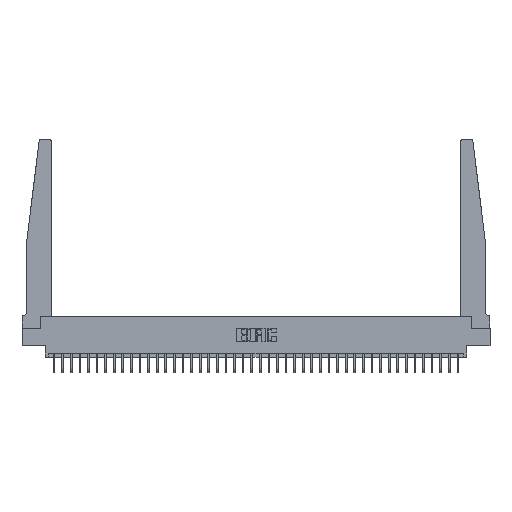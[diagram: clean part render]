
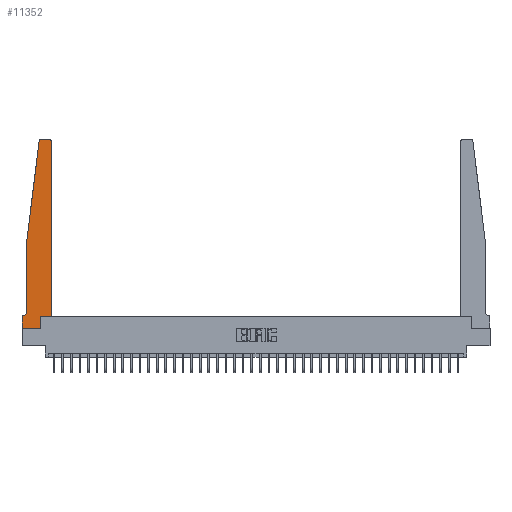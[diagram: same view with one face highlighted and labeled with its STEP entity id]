
A CAD part, top view. The second image highlights one B-rep face of the part: STEP entity #11352.
In plain terms, the highlighted planar face has unit normal (0, 0, 1).
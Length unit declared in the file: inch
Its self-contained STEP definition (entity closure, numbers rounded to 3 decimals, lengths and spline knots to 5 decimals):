
#460 = CARTESIAN_POINT ( 'NONE',  ( 0.425, 2.72, 0.37 ) ) ;
#1058 = EDGE_LOOP ( 'NONE', ( #14955, #33031, #28609, #17216, #21894, #33223, #4994, #19505, #8686, #12310, #12624, #16749 ) ) ;
#1568 = VERTEX_POINT ( 'NONE', #8934 ) ;
#1722 = LINE ( 'NONE', #28738, #21538 ) ;
#2375 = DIRECTION ( 'NONE',  ( 1., 0., 0. ) ) ;
#2389 = LINE ( 'NONE', #35909, #11811 ) ;
#3018 = CARTESIAN_POINT ( 'NONE',  ( 0.24675, 2.72367, 0.37 ) ) ;
#3846 = CARTESIAN_POINT ( 'NONE',  ( 0.015, 0.2375, 0.37 ) ) ;
#4205 = VECTOR ( 'NONE', #15173, 39.37008 ) ;
#4994 = ORIENTED_EDGE ( 'NONE', *, *, #14231, .T. ) ;
#5200 = VERTEX_POINT ( 'NONE', #8440 ) ;
#6178 = AXIS2_PLACEMENT_3D ( 'NONE', #28668, #14218, #34737 ) ;
#6329 = DIRECTION ( 'NONE',  ( 0., 1., 0. ) ) ;
#6392 = EDGE_CURVE ( 'NONE', #35005, #17127, #34311, .T. ) ;
#6412 = DIRECTION ( 'NONE',  ( 1., 0., 0. ) ) ;
#6859 = PLANE ( 'NONE',  #18879 ) ;
#7048 = DIRECTION ( 'NONE',  ( -1., 0., 0. ) ) ;
#7368 = DIRECTION ( 'NONE',  ( -0.122, -0.992, 0. ) ) ;
#7501 = CARTESIAN_POINT ( 'NONE',  ( 0.2605, 0., 0.37 ) ) ;
#7635 = EDGE_CURVE ( 'NONE', #17127, #5200, #26704, .T. ) ;
#7813 = VERTEX_POINT ( 'NONE', #18453 ) ;
#7896 = DIRECTION ( 'NONE',  ( 1., 0., 0. ) ) ;
#7900 = VERTEX_POINT ( 'NONE', #30471 ) ;
#8000 = DIRECTION ( 'NONE',  ( 0., 0., 1. ) ) ;
#8421 = VERTEX_POINT ( 'NONE', #22709 ) ;
#8440 = CARTESIAN_POINT ( 'NONE',  ( 0.2605, 0.18, 0.37 ) ) ;
#8665 = CIRCLE ( 'NONE', #6178, 0.03 ) ;
#8686 = ORIENTED_EDGE ( 'NONE', *, *, #7635, .T. ) ;
#8934 = CARTESIAN_POINT ( 'NONE',  ( 0.065, 1.25, 0.37 ) ) ;
#9943 = CARTESIAN_POINT ( 'NONE',  ( 0.425, 0.18, 0.37 ) ) ;
#10361 = DIRECTION ( 'NONE',  ( -1., 0., 0. ) ) ;
#11352 = ADVANCED_FACE ( 'NONE', ( #17073 ), #6859, .T. ) ;
#11811 = VECTOR ( 'NONE', #36038, 39.37008 ) ;
#12098 = CARTESIAN_POINT ( 'NONE',  ( 0.2605, 0.18, 0.37 ) ) ;
#12310 = ORIENTED_EDGE ( 'NONE', *, *, #14349, .T. ) ;
#12624 = ORIENTED_EDGE ( 'NONE', *, *, #32546, .T. ) ;
#12666 = EDGE_CURVE ( 'NONE', #19054, #1568, #15194, .T. ) ;
#12668 = DIRECTION ( 'NONE',  ( 0., 0., 1. ) ) ;
#13030 = CARTESIAN_POINT ( 'NONE',  ( 0.065, 1.25, 0.37 ) ) ;
#13036 = VECTOR ( 'NONE', #7048, 39.37008 ) ;
#13318 = DIRECTION ( 'NONE',  ( 0., -1., 0. ) ) ;
#13451 = DIRECTION ( 'NONE',  ( -1., 0., 0. ) ) ;
#13858 = EDGE_CURVE ( 'NONE', #1568, #29915, #29401, .T. ) ;
#13913 = EDGE_CURVE ( 'NONE', #15332, #27472, #32586, .T. ) ;
#14218 = DIRECTION ( 'NONE',  ( 0., 0., 1. ) ) ;
#14231 = EDGE_CURVE ( 'NONE', #7813, #35005, #2389, .T. ) ;
#14349 = EDGE_CURVE ( 'NONE', #5200, #17589, #17257, .T. ) ;
#14556 = VECTOR ( 'NONE', #13318, 39.37008 ) ;
#14955 = ORIENTED_EDGE ( 'NONE', *, *, #31539, .T. ) ;
#15173 = DIRECTION ( 'NONE',  ( 1., 0., 0. ) ) ;
#15194 = LINE ( 'NONE', #13030, #37229 ) ;
#15332 = VERTEX_POINT ( 'NONE', #460 ) ;
#16749 = ORIENTED_EDGE ( 'NONE', *, *, #13913, .T. ) ;
#17073 = FACE_OUTER_BOUND ( 'NONE', #1058, .T. ) ;
#17127 = VERTEX_POINT ( 'NONE', #7501 ) ;
#17216 = ORIENTED_EDGE ( 'NONE', *, *, #13858, .T. ) ;
#17257 = LINE ( 'NONE', #9943, #4205 ) ;
#17589 = VERTEX_POINT ( 'NONE', #20838 ) ;
#18207 = DIRECTION ( 'NONE',  ( 0., 0., -1. ) ) ;
#18453 = CARTESIAN_POINT ( 'NONE',  ( 0., 0.1875, 0.37 ) ) ;
#18879 = AXIS2_PLACEMENT_3D ( 'NONE', #24354, #12668, #6412 ) ;
#19054 = VERTEX_POINT ( 'NONE', #3018 ) ;
#19081 = EDGE_CURVE ( 'NONE', #8421, #19054, #8665, .T. ) ;
#19505 = ORIENTED_EDGE ( 'NONE', *, *, #6392, .T. ) ;
#19626 = AXIS2_PLACEMENT_3D ( 'NONE', #31179, #8000, #2375 ) ;
#20141 = AXIS2_PLACEMENT_3D ( 'NONE', #3846, #18207, #10361 ) ;
#20838 = CARTESIAN_POINT ( 'NONE',  ( 0.425, 0.18, 0.37 ) ) ;
#21330 = VECTOR ( 'NONE', #6329, 39.37008 ) ;
#21538 = VECTOR ( 'NONE', #32160, 39.37008 ) ;
#21894 = ORIENTED_EDGE ( 'NONE', *, *, #30937, .T. ) ;
#22709 = CARTESIAN_POINT ( 'NONE',  ( 0.27653, 2.75, 0.37 ) ) ;
#24354 = CARTESIAN_POINT ( 'NONE',  ( 0., 0.1875, 0.37 ) ) ;
#25540 = CARTESIAN_POINT ( 'NONE',  ( 0.395, 2.75, 0.37 ) ) ;
#26612 = LINE ( 'NONE', #33235, #27974 ) ;
#26704 = LINE ( 'NONE', #12098, #21330 ) ;
#27295 = VECTOR ( 'NONE', #7896, 39.37008 ) ;
#27472 = VERTEX_POINT ( 'NONE', #25540 ) ;
#27804 = CARTESIAN_POINT ( 'NONE',  ( 0., 0., 0.37 ) ) ;
#27974 = VECTOR ( 'NONE', #13451, 39.37008 ) ;
#28454 = CARTESIAN_POINT ( 'NONE',  ( 0., 0., 0.37 ) ) ;
#28609 = ORIENTED_EDGE ( 'NONE', *, *, #12666, .T. ) ;
#28668 = CARTESIAN_POINT ( 'NONE',  ( 0.27653, 2.72, 0.37 ) ) ;
#28738 = CARTESIAN_POINT ( 'NONE',  ( 0.425, 0.18, 0.37 ) ) ;
#29401 = LINE ( 'NONE', #33737, #14556 ) ;
#29915 = VERTEX_POINT ( 'NONE', #36133 ) ;
#30471 = CARTESIAN_POINT ( 'NONE',  ( 0.015, 0.1875, 0.37 ) ) ;
#30937 = EDGE_CURVE ( 'NONE', #29915, #7900, #31135, .T. ) ;
#31135 = CIRCLE ( 'NONE', #20141, 0.05 ) ;
#31179 = CARTESIAN_POINT ( 'NONE',  ( 0.395, 2.72, 0.37 ) ) ;
#31539 = EDGE_CURVE ( 'NONE', #27472, #8421, #35604, .T. ) ;
#32160 = DIRECTION ( 'NONE',  ( 0., 1., 0. ) ) ;
#32546 = EDGE_CURVE ( 'NONE', #17589, #15332, #1722, .T. ) ;
#32586 = CIRCLE ( 'NONE', #19626, 0.03 ) ;
#33031 = ORIENTED_EDGE ( 'NONE', *, *, #19081, .T. ) ;
#33223 = ORIENTED_EDGE ( 'NONE', *, *, #36788, .T. ) ;
#33235 = CARTESIAN_POINT ( 'NONE',  ( 0.065, 0.1875, 0.37 ) ) ;
#33737 = CARTESIAN_POINT ( 'NONE',  ( 0.065, 1.25, 0.37 ) ) ;
#34311 = LINE ( 'NONE', #27804, #27295 ) ;
#34737 = DIRECTION ( 'NONE',  ( 1., 0., 0. ) ) ;
#35005 = VERTEX_POINT ( 'NONE', #28454 ) ;
#35394 = CARTESIAN_POINT ( 'NONE',  ( 0.25, 2.75, 0.37 ) ) ;
#35604 = LINE ( 'NONE', #35394, #13036 ) ;
#35909 = CARTESIAN_POINT ( 'NONE',  ( 0., 0., 0.37 ) ) ;
#36038 = DIRECTION ( 'NONE',  ( 0., -1., 0. ) ) ;
#36133 = CARTESIAN_POINT ( 'NONE',  ( 0.065, 0.2375, 0.37 ) ) ;
#36788 = EDGE_CURVE ( 'NONE', #7900, #7813, #26612, .T. ) ;
#37229 = VECTOR ( 'NONE', #7368, 39.37008 ) ;
